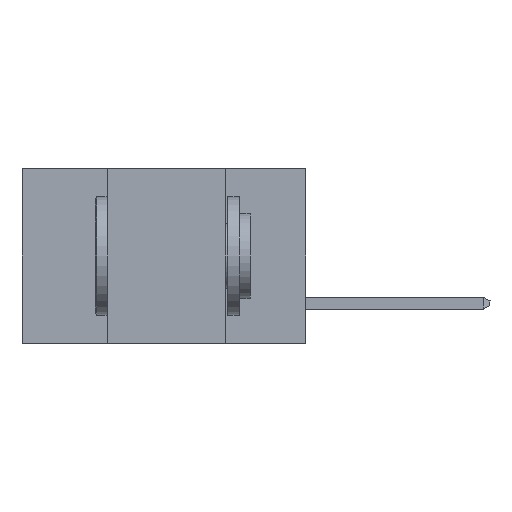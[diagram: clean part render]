
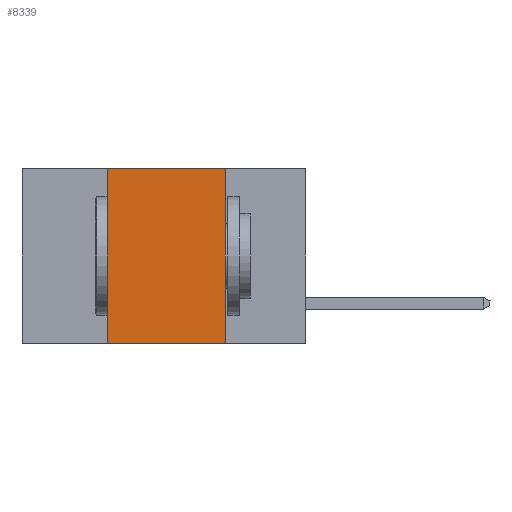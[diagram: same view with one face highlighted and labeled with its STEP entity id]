
A CAD part, left-side view. The second image highlights one B-rep face of the part: STEP entity #8339.
In plain terms, the highlighted planar face has unit normal (-1, 0, 0).
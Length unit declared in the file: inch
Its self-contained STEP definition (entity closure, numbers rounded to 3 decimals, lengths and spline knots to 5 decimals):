
#639 = ORIENTED_EDGE ( 'NONE', *, *, #3866, .T. ) ;
#653 = VECTOR ( 'NONE', #17832, 39.37008 ) ;
#2126 = AXIS2_PLACEMENT_3D ( 'NONE', #8140, #15106, #3850 ) ;
#2217 = PLANE ( 'NONE',  #2126 ) ;
#2827 = VECTOR ( 'NONE', #4251, 39.37008 ) ;
#2838 = DIRECTION ( 'NONE',  ( 0., -1., 0. ) ) ;
#3465 = ORIENTED_EDGE ( 'NONE', *, *, #12921, .F. ) ;
#3812 = VECTOR ( 'NONE', #2838, 39.37008 ) ;
#3850 = DIRECTION ( 'NONE',  ( 0., 0., -1. ) ) ;
#3866 = EDGE_CURVE ( 'NONE', #15437, #8432, #15798, .T. ) ;
#4251 = DIRECTION ( 'NONE',  ( 0., -1., 0. ) ) ;
#4432 = DIRECTION ( 'NONE',  ( 0., 0., 1. ) ) ;
#5599 = CARTESIAN_POINT ( 'NONE',  ( 0., 0.42, 0. ) ) ;
#7309 = CARTESIAN_POINT ( 'NONE',  ( 0., 0.42, 0. ) ) ;
#7745 = ORIENTED_EDGE ( 'NONE', *, *, #14304, .F. ) ;
#8140 = CARTESIAN_POINT ( 'NONE',  ( 0., 0.6, 0. ) ) ;
#8339 = ADVANCED_FACE ( 'NONE', ( #10070 ), #2217, .F. ) ;
#8432 = VERTEX_POINT ( 'NONE', #12878 ) ;
#10070 = FACE_OUTER_BOUND ( 'NONE', #10958, .T. ) ;
#10958 = EDGE_LOOP ( 'NONE', ( #13389, #7745, #3465, #639 ) ) ;
#11404 = CARTESIAN_POINT ( 'NONE',  ( 0., 0.6, 0. ) ) ;
#11850 = VERTEX_POINT ( 'NONE', #15216 ) ;
#12507 = VERTEX_POINT ( 'NONE', #7309 ) ;
#12531 = LINE ( 'NONE', #16595, #653 ) ;
#12878 = CARTESIAN_POINT ( 'NONE',  ( 0., 0.17, -0.37 ) ) ;
#12921 = EDGE_CURVE ( 'NONE', #15437, #12507, #17932, .T. ) ;
#13389 = ORIENTED_EDGE ( 'NONE', *, *, #15864, .F. ) ;
#14164 = VECTOR ( 'NONE', #4432, 39.37008 ) ;
#14304 = EDGE_CURVE ( 'NONE', #12507, #11850, #14771, .T. ) ;
#14439 = CARTESIAN_POINT ( 'NONE',  ( 0., 0.6, -0.37 ) ) ;
#14771 = LINE ( 'NONE', #11404, #3812 ) ;
#15106 = DIRECTION ( 'NONE',  ( 1., 0., 0. ) ) ;
#15216 = CARTESIAN_POINT ( 'NONE',  ( 0., 0.17, 0. ) ) ;
#15437 = VERTEX_POINT ( 'NONE', #18335 ) ;
#15798 = LINE ( 'NONE', #14439, #2827 ) ;
#15864 = EDGE_CURVE ( 'NONE', #11850, #8432, #12531, .T. ) ;
#16595 = CARTESIAN_POINT ( 'NONE',  ( 0., 0.17, 0. ) ) ;
#17832 = DIRECTION ( 'NONE',  ( 0., 0., -1. ) ) ;
#17932 = LINE ( 'NONE', #5599, #14164 ) ;
#18335 = CARTESIAN_POINT ( 'NONE',  ( 0., 0.42, -0.37 ) ) ;
